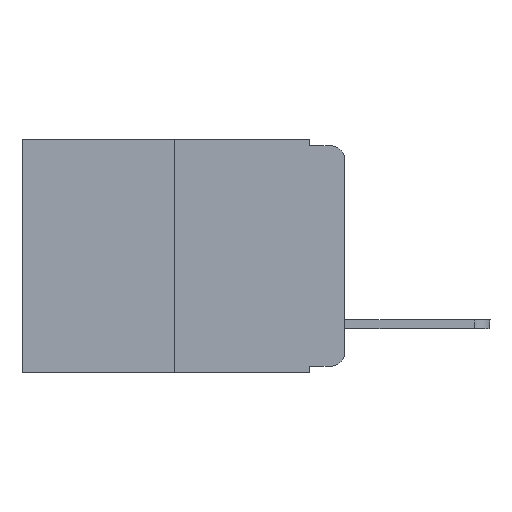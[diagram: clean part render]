
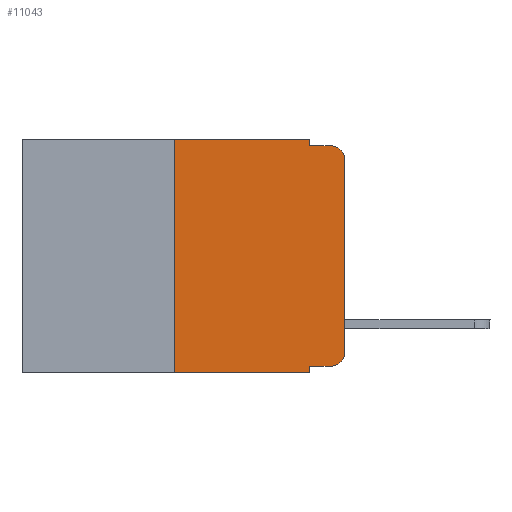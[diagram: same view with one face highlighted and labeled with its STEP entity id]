
A CAD part, left-side view. The second image highlights one B-rep face of the part: STEP entity #11043.
In plain terms, the highlighted planar face has unit normal (-1, 0, 0).
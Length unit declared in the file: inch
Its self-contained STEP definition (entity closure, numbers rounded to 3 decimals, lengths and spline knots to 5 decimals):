
#256 = DIRECTION ( 'NONE',  ( 0., 0., -1. ) ) ;
#319 = VERTEX_POINT ( 'NONE', #12830 ) ;
#352 = VECTOR ( 'NONE', #3490, 39.37008 ) ;
#480 = DIRECTION ( 'NONE',  ( 0., 0., -1. ) ) ;
#688 = VERTEX_POINT ( 'NONE', #7361 ) ;
#734 = VERTEX_POINT ( 'NONE', #7412 ) ;
#827 = VECTOR ( 'NONE', #256, 39.37008 ) ;
#1012 = VECTOR ( 'NONE', #10310, 39.37008 ) ;
#1106 = ORIENTED_EDGE ( 'NONE', *, *, #8341, .F. ) ;
#1244 = VECTOR ( 'NONE', #15051, 39.37008 ) ;
#1335 = AXIS2_PLACEMENT_3D ( 'NONE', #9095, #14011, #15095 ) ;
#1350 = ORIENTED_EDGE ( 'NONE', *, *, #3870, .T. ) ;
#1557 = CARTESIAN_POINT ( 'NONE',  ( 0., 0.051, -0.333 ) ) ;
#1698 = CARTESIAN_POINT ( 'NONE',  ( 0., 0.051, -0.333 ) ) ;
#1954 = CARTESIAN_POINT ( 'NONE',  ( 0., 0.051, -0.01 ) ) ;
#2267 = ORIENTED_EDGE ( 'NONE', *, *, #11453, .F. ) ;
#2720 = EDGE_CURVE ( 'NONE', #9867, #319, #2803, .T. ) ;
#2803 = LINE ( 'NONE', #1557, #1244 ) ;
#2889 = ORIENTED_EDGE ( 'NONE', *, *, #6693, .T. ) ;
#3490 = DIRECTION ( 'NONE',  ( 0., -1., 0. ) ) ;
#3572 = FACE_OUTER_BOUND ( 'NONE', #5624, .T. ) ;
#3870 = EDGE_CURVE ( 'NONE', #688, #6680, #14855, .T. ) ;
#4076 = LINE ( 'NONE', #12419, #827 ) ;
#4128 = DIRECTION ( 'NONE',  ( -1., 0., 0. ) ) ;
#4619 = EDGE_CURVE ( 'NONE', #9867, #6484, #4076, .T. ) ;
#4839 = VERTEX_POINT ( 'NONE', #1954 ) ;
#4896 = VERTEX_POINT ( 'NONE', #14439 ) ;
#5088 = LINE ( 'NONE', #9680, #11224 ) ;
#5340 = CARTESIAN_POINT ( 'NONE',  ( 0., 0.02, -0.01 ) ) ;
#5624 = EDGE_LOOP ( 'NONE', ( #13219, #1350, #15887, #2267, #1106, #12103, #9777, #11817, #12164, #2889 ) ) ;
#5937 = CIRCLE ( 'NONE', #1335, 0.02 ) ;
#6112 = EDGE_CURVE ( 'NONE', #4896, #688, #8261, .T. ) ;
#6213 = CARTESIAN_POINT ( 'NONE',  ( 0., 0.051, 0. ) ) ;
#6484 = VERTEX_POINT ( 'NONE', #11240 ) ;
#6540 = PLANE ( 'NONE',  #12157 ) ;
#6608 = CARTESIAN_POINT ( 'NONE',  ( 0., 0.02, -0.03 ) ) ;
#6680 = VERTEX_POINT ( 'NONE', #5340 ) ;
#6693 = EDGE_CURVE ( 'NONE', #319, #4896, #5937, .T. ) ;
#7180 = DIRECTION ( 'NONE',  ( 0., 0., -1. ) ) ;
#7361 = CARTESIAN_POINT ( 'NONE',  ( 0., 0., -0.03 ) ) ;
#7412 = CARTESIAN_POINT ( 'NONE',  ( 0., 0.25, 0. ) ) ;
#7691 = LINE ( 'NONE', #8439, #13807 ) ;
#8261 = LINE ( 'NONE', #11724, #10543 ) ;
#8341 = EDGE_CURVE ( 'NONE', #734, #11538, #7691, .T. ) ;
#8365 = CARTESIAN_POINT ( 'NONE',  ( 0., 0.473, -0.343 ) ) ;
#8439 = CARTESIAN_POINT ( 'NONE',  ( 0., 0.473, 0. ) ) ;
#8616 = VECTOR ( 'NONE', #10842, 39.37008 ) ;
#8803 = DIRECTION ( 'NONE',  ( 0., 0., -1. ) ) ;
#9095 = CARTESIAN_POINT ( 'NONE',  ( 0., 0.02, -0.313 ) ) ;
#9680 = CARTESIAN_POINT ( 'NONE',  ( 0., 0.051, 0. ) ) ;
#9777 = ORIENTED_EDGE ( 'NONE', *, *, #15856, .T. ) ;
#9867 = VERTEX_POINT ( 'NONE', #1698 ) ;
#10310 = DIRECTION ( 'NONE',  ( 0., -1., 0. ) ) ;
#10543 = VECTOR ( 'NONE', #15257, 39.37008 ) ;
#10842 = DIRECTION ( 'NONE',  ( 0., 0., 1. ) ) ;
#11043 = ADVANCED_FACE ( 'NONE', ( #3572 ), #6540, .F. ) ;
#11224 = VECTOR ( 'NONE', #7180, 39.37008 ) ;
#11240 = CARTESIAN_POINT ( 'NONE',  ( 0., 0.051, -0.343 ) ) ;
#11271 = AXIS2_PLACEMENT_3D ( 'NONE', #6608, #4128, #8803 ) ;
#11276 = LINE ( 'NONE', #8365, #352 ) ;
#11453 = EDGE_CURVE ( 'NONE', #11538, #4839, #5088, .T. ) ;
#11538 = VERTEX_POINT ( 'NONE', #6213 ) ;
#11719 = VERTEX_POINT ( 'NONE', #12733 ) ;
#11724 = CARTESIAN_POINT ( 'NONE',  ( 0., 0., 0. ) ) ;
#11817 = ORIENTED_EDGE ( 'NONE', *, *, #4619, .F. ) ;
#12103 = ORIENTED_EDGE ( 'NONE', *, *, #15318, .F. ) ;
#12136 = DIRECTION ( 'NONE',  ( 0., -1., 0. ) ) ;
#12157 = AXIS2_PLACEMENT_3D ( 'NONE', #13703, #14121, #480 ) ;
#12164 = ORIENTED_EDGE ( 'NONE', *, *, #2720, .T. ) ;
#12419 = CARTESIAN_POINT ( 'NONE',  ( 0., 0.051, 0. ) ) ;
#12733 = CARTESIAN_POINT ( 'NONE',  ( 0., 0.25, -0.343 ) ) ;
#12830 = CARTESIAN_POINT ( 'NONE',  ( 0., 0.02, -0.333 ) ) ;
#13219 = ORIENTED_EDGE ( 'NONE', *, *, #6112, .T. ) ;
#13433 = EDGE_CURVE ( 'NONE', #4839, #6680, #14607, .T. ) ;
#13584 = LINE ( 'NONE', #15866, #8616 ) ;
#13703 = CARTESIAN_POINT ( 'NONE',  ( 0., 0.473, 0. ) ) ;
#13807 = VECTOR ( 'NONE', #12136, 39.37008 ) ;
#14011 = DIRECTION ( 'NONE',  ( -1., 0., 0. ) ) ;
#14121 = DIRECTION ( 'NONE',  ( 1., 0., 0. ) ) ;
#14439 = CARTESIAN_POINT ( 'NONE',  ( 0., 0., -0.313 ) ) ;
#14607 = LINE ( 'NONE', #15338, #1012 ) ;
#14855 = CIRCLE ( 'NONE', #11271, 0.02 ) ;
#15051 = DIRECTION ( 'NONE',  ( 0., -1., 0. ) ) ;
#15095 = DIRECTION ( 'NONE',  ( 0., 0., -1. ) ) ;
#15257 = DIRECTION ( 'NONE',  ( 0., 0., 1. ) ) ;
#15318 = EDGE_CURVE ( 'NONE', #11719, #734, #13584, .T. ) ;
#15338 = CARTESIAN_POINT ( 'NONE',  ( 0., 0.051, -0.01 ) ) ;
#15856 = EDGE_CURVE ( 'NONE', #11719, #6484, #11276, .T. ) ;
#15866 = CARTESIAN_POINT ( 'NONE',  ( 0., 0.25, 0. ) ) ;
#15887 = ORIENTED_EDGE ( 'NONE', *, *, #13433, .F. ) ;
